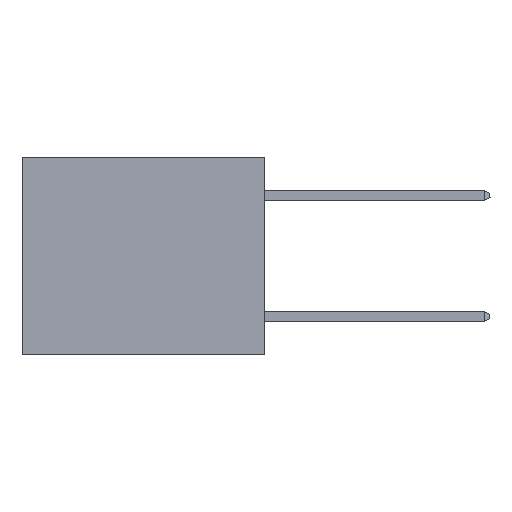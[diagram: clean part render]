
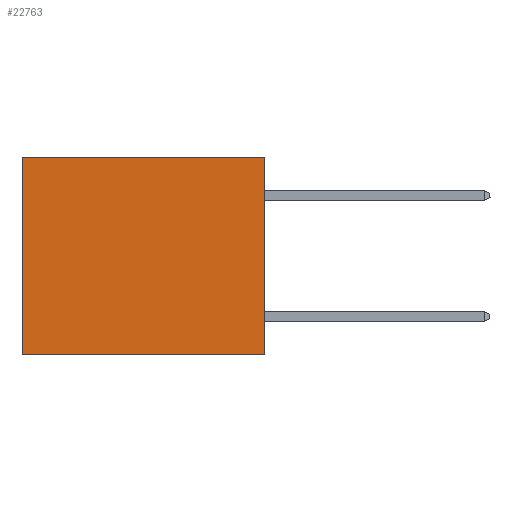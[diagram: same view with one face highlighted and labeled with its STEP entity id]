
A CAD part, left-side view. The second image highlights one B-rep face of the part: STEP entity #22763.
In plain terms, the highlighted planar face has unit normal (-1, 0, 0).
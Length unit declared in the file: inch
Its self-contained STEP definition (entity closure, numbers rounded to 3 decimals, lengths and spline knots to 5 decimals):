
#1554 = DIRECTION ( 'NONE',  ( 0., 1., 0. ) ) ;
#1928 = VECTOR ( 'NONE', #14225, 39.37008 ) ;
#2048 = ORIENTED_EDGE ( 'NONE', *, *, #8176, .T. ) ;
#3965 = PLANE ( 'NONE',  #8929 ) ;
#4587 = DIRECTION ( 'NONE',  ( 0., 0., -1. ) ) ;
#5380 = ORIENTED_EDGE ( 'NONE', *, *, #7140, .T. ) ;
#5679 = LINE ( 'NONE', #19455, #13487 ) ;
#5793 = CARTESIAN_POINT ( 'NONE',  ( 0.3165, 0., -0.49 ) ) ;
#5832 = ORIENTED_EDGE ( 'NONE', *, *, #9545, .F. ) ;
#6009 = EDGE_LOOP ( 'NONE', ( #5380, #20236, #5832, #2048 ) ) ;
#6605 = VECTOR ( 'NONE', #10788, 39.37008 ) ;
#6799 = EDGE_CURVE ( 'NONE', #8000, #10924, #19392, .T. ) ;
#7140 = EDGE_CURVE ( 'NONE', #11002, #10924, #9660, .T. ) ;
#7880 = CARTESIAN_POINT ( 'NONE',  ( 0.3165, 0., 0. ) ) ;
#8000 = VERTEX_POINT ( 'NONE', #12014 ) ;
#8176 = EDGE_CURVE ( 'NONE', #16464, #11002, #5679, .T. ) ;
#8929 = AXIS2_PLACEMENT_3D ( 'NONE', #5793, #21908, #14833 ) ;
#9545 = EDGE_CURVE ( 'NONE', #16464, #8000, #10091, .T. ) ;
#9660 = LINE ( 'NONE', #20633, #17719 ) ;
#10091 = LINE ( 'NONE', #12411, #1928 ) ;
#10788 = DIRECTION ( 'NONE',  ( 0., 1., 0. ) ) ;
#10924 = VERTEX_POINT ( 'NONE', #19619 ) ;
#11002 = VERTEX_POINT ( 'NONE', #22285 ) ;
#12014 = CARTESIAN_POINT ( 'NONE',  ( 0.3165, 0., -0.49 ) ) ;
#12411 = CARTESIAN_POINT ( 'NONE',  ( 0.3165, 0., -0.49 ) ) ;
#13487 = VECTOR ( 'NONE', #1554, 39.37008 ) ;
#14225 = DIRECTION ( 'NONE',  ( 0., 0., -1. ) ) ;
#14833 = DIRECTION ( 'NONE',  ( 0., 0., -1. ) ) ;
#16464 = VERTEX_POINT ( 'NONE', #7880 ) ;
#17719 = VECTOR ( 'NONE', #4587, 39.37008 ) ;
#19392 = LINE ( 'NONE', #19578, #6605 ) ;
#19455 = CARTESIAN_POINT ( 'NONE',  ( 0.3165, 0., 0. ) ) ;
#19578 = CARTESIAN_POINT ( 'NONE',  ( 0.3165, 0., -0.49 ) ) ;
#19619 = CARTESIAN_POINT ( 'NONE',  ( 0.3165, 0.6, -0.49 ) ) ;
#20236 = ORIENTED_EDGE ( 'NONE', *, *, #6799, .F. ) ;
#20633 = CARTESIAN_POINT ( 'NONE',  ( 0.3165, 0.6, -0.49 ) ) ;
#21908 = DIRECTION ( 'NONE',  ( 1., 0., 0. ) ) ;
#21954 = FACE_OUTER_BOUND ( 'NONE', #6009, .T. ) ;
#22285 = CARTESIAN_POINT ( 'NONE',  ( 0.3165, 0.6, 0. ) ) ;
#22763 = ADVANCED_FACE ( 'NONE', ( #21954 ), #3965, .F. ) ;
